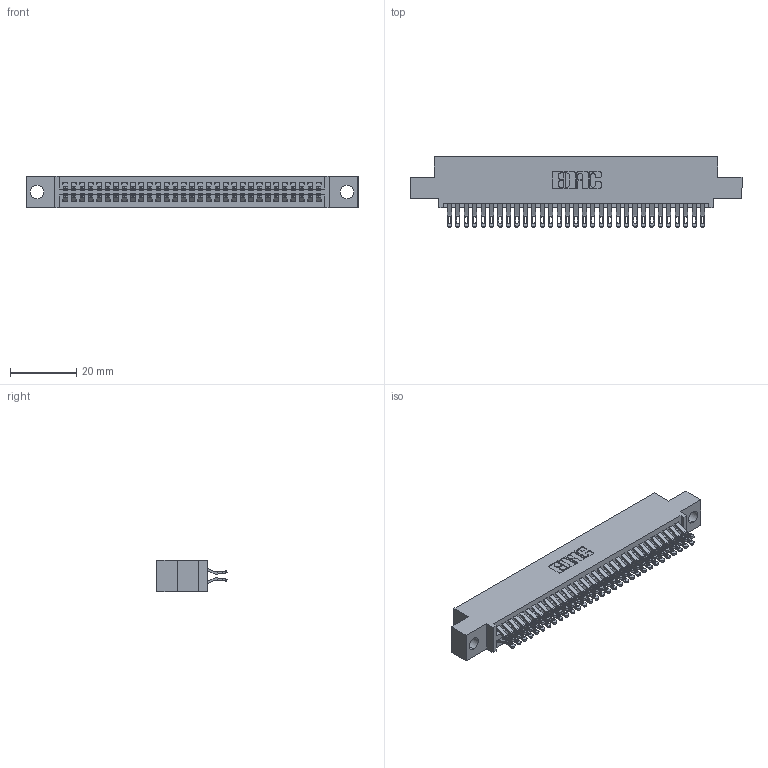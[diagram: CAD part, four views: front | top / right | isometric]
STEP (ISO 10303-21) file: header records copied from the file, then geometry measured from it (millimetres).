
FILE_DESCRIPTION (( 'STEP AP203' ), '1' );
FILE_NAME ('345-062-555-504.STEP', '2021-05-20T06:14:44', ( '' ), ( '' ), 'SwSTEP 2.0', 'SolidWorks 2020', '' );
FILE_SCHEMA (( 'CONFIG_CONTROL_DESIGN' ));
Length unit declared in the file: inch
Products named in the file (3): 345-062-555-504; 345 Part_0.110 Offset - 0.156 Dia-TI; 345-292-001_555 Tail
Assembly tree (63 placements, depth 2):
  345-062-555-504
    345 Part_0.110 Offset - 0.156 Dia-TI
    345-292-001_555 Tail  x62
Bounding box: 99.95 x 21.13 x 9.4 mm (x, y, z)
Volume: 9607.6 mm3; surface area: 14558.5 mm2
Topology: 63 solids, 63 shells, 3616 faces, 11363 edges, 7574 vertices
Faces by surface type: plane 2020, cylinder 1596
Entity records: 26681 total; most frequent: CARTESIAN_POINT 4524, ORIENTED_EDGE 4426, DIRECTION 3969, EDGE_CURVE 2213, VECTOR 1937, LINE 1937, VERTEX_POINT 1474, AXIS2_PLACEMENT_3D 1016
